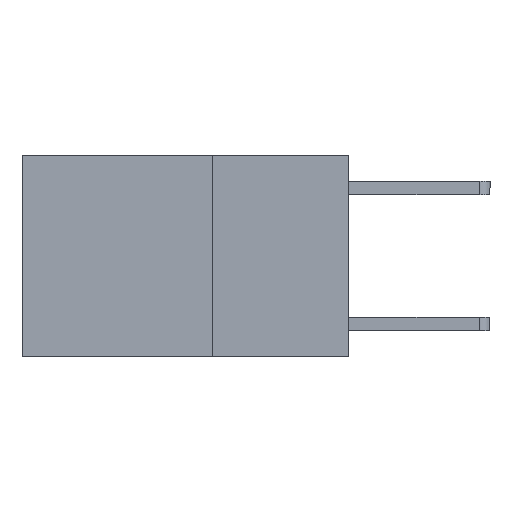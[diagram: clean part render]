
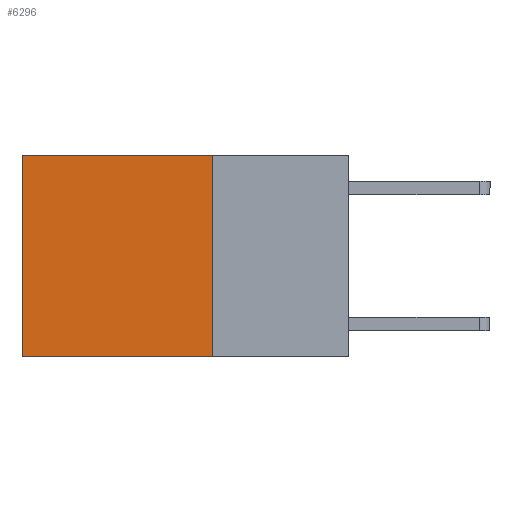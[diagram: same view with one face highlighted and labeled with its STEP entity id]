
A CAD part, left-side view. The second image highlights one B-rep face of the part: STEP entity #6296.
In plain terms, the highlighted planar face has unit normal (-1, 0, 0).
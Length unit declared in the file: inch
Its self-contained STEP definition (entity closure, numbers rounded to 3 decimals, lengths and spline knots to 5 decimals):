
#33 = CARTESIAN_POINT ( 'NONE',  ( 0.2625, 0.6, 0. ) ) ;
#381 = ORIENTED_EDGE ( 'NONE', *, *, #2536, .F. ) ;
#599 = VERTEX_POINT ( 'NONE', #8554 ) ;
#600 = CARTESIAN_POINT ( 'NONE',  ( 0.2625, 0.25, -0.37 ) ) ;
#641 = LINE ( 'NONE', #600, #2674 ) ;
#940 = CARTESIAN_POINT ( 'NONE',  ( 0.2625, 0.25, 0. ) ) ;
#1058 = VERTEX_POINT ( 'NONE', #33 ) ;
#1257 = DIRECTION ( 'NONE',  ( 0., 1., 0. ) ) ;
#1290 = DIRECTION ( 'NONE',  ( 0., 1., 0. ) ) ;
#1592 = DIRECTION ( 'NONE',  ( 1., 0., 0. ) ) ;
#2039 = EDGE_CURVE ( 'NONE', #3768, #1058, #6701, .T. ) ;
#2242 = CARTESIAN_POINT ( 'NONE',  ( 0.2625, 0.25, 0. ) ) ;
#2349 = VECTOR ( 'NONE', #1257, 39.37008 ) ;
#2536 = EDGE_CURVE ( 'NONE', #599, #5003, #641, .T. ) ;
#2674 = VECTOR ( 'NONE', #1290, 39.37008 ) ;
#2683 = CARTESIAN_POINT ( 'NONE',  ( 0.2625, 0.25, 0. ) ) ;
#3007 = EDGE_LOOP ( 'NONE', ( #7062, #381, #7857, #4489 ) ) ;
#3486 = CARTESIAN_POINT ( 'NONE',  ( 0.2625, 0.6, -0.37 ) ) ;
#3588 = FACE_OUTER_BOUND ( 'NONE', #3007, .T. ) ;
#3768 = VERTEX_POINT ( 'NONE', #2242 ) ;
#3891 = AXIS2_PLACEMENT_3D ( 'NONE', #4954, #1592, #4288 ) ;
#4113 = PLANE ( 'NONE',  #3891 ) ;
#4288 = DIRECTION ( 'NONE',  ( 0., 0., -1. ) ) ;
#4485 = DIRECTION ( 'NONE',  ( 0., 0., -1. ) ) ;
#4489 = ORIENTED_EDGE ( 'NONE', *, *, #2039, .T. ) ;
#4954 = CARTESIAN_POINT ( 'NONE',  ( 0.2625, 0.25, 0. ) ) ;
#4999 = LINE ( 'NONE', #940, #7105 ) ;
#5003 = VERTEX_POINT ( 'NONE', #3486 ) ;
#6296 = ADVANCED_FACE ( 'NONE', ( #3588 ), #4113, .F. ) ;
#6333 = DIRECTION ( 'NONE',  ( 0., 0., -1. ) ) ;
#6517 = LINE ( 'NONE', #7216, #6904 ) ;
#6701 = LINE ( 'NONE', #2683, #2349 ) ;
#6827 = EDGE_CURVE ( 'NONE', #1058, #5003, #6517, .T. ) ;
#6904 = VECTOR ( 'NONE', #4485, 39.37008 ) ;
#7062 = ORIENTED_EDGE ( 'NONE', *, *, #6827, .T. ) ;
#7105 = VECTOR ( 'NONE', #6333, 39.37008 ) ;
#7216 = CARTESIAN_POINT ( 'NONE',  ( 0.2625, 0.6, 0. ) ) ;
#7609 = EDGE_CURVE ( 'NONE', #3768, #599, #4999, .T. ) ;
#7857 = ORIENTED_EDGE ( 'NONE', *, *, #7609, .F. ) ;
#8554 = CARTESIAN_POINT ( 'NONE',  ( 0.2625, 0.25, -0.37 ) ) ;
